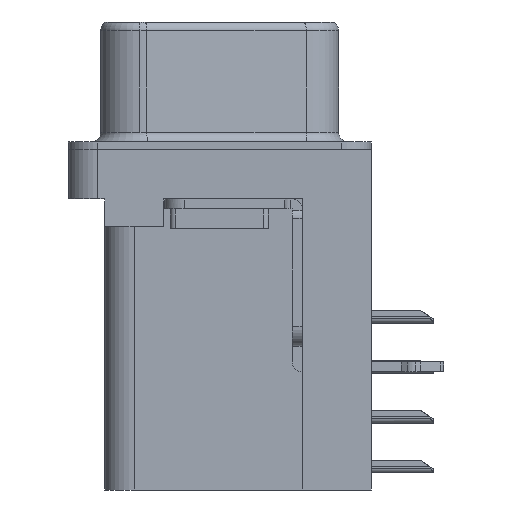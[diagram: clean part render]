
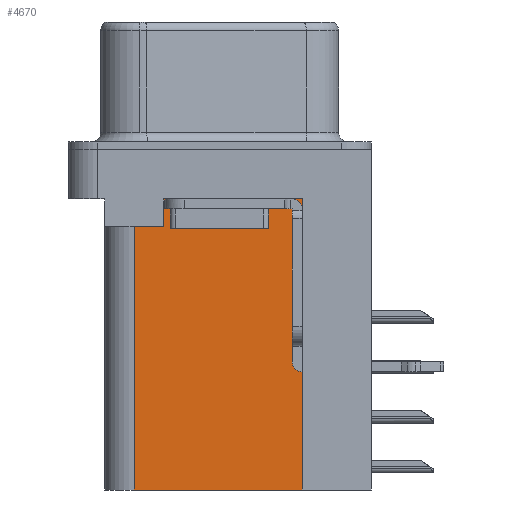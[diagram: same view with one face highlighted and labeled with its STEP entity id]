
A CAD part, left-side view. The second image highlights one B-rep face of the part: STEP entity #4670.
In plain terms, the highlighted planar face has unit normal (-1, 0, 0).
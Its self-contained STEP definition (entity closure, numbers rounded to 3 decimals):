
#1924 = EDGE_CURVE ( 'NONE', #36063, #21664, #15045, .T. ) ;
#2300 = LINE ( 'NONE', #3465, #17706 ) ;
#2521 = DIRECTION ( 'NONE',  ( 0., 1., 0. ) ) ;
#2881 = VERTEX_POINT ( 'NONE', #8026 ) ;
#3465 = CARTESIAN_POINT ( 'NONE',  ( 3.75, 4.35, -17.3 ) ) ;
#4670 = ADVANCED_FACE ( 'NONE', ( #11981 ), #25382, .F. ) ;
#5185 = DIRECTION ( 'NONE',  ( 0., 0., -1. ) ) ;
#5504 = VECTOR ( 'NONE', #10067, 1000. ) ;
#5625 = ORIENTED_EDGE ( 'NONE', *, *, #34127, .F. ) ;
#6606 = VECTOR ( 'NONE', #33735, 1000. ) ;
#7624 = ORIENTED_EDGE ( 'NONE', *, *, #16834, .T. ) ;
#8026 = CARTESIAN_POINT ( 'NONE',  ( 3.75, 2.85, -3.9 ) ) ;
#8383 = VERTEX_POINT ( 'NONE', #8876 ) ;
#8876 = CARTESIAN_POINT ( 'NONE',  ( 3.75, 4.35, -3.9 ) ) ;
#9161 = CARTESIAN_POINT ( 'NONE',  ( 3.75, 0., -3.9 ) ) ;
#9656 = CARTESIAN_POINT ( 'NONE',  ( 3.75, 4.35, -17.3 ) ) ;
#10067 = DIRECTION ( 'NONE',  ( 0., 0., 1. ) ) ;
#10268 = LINE ( 'NONE', #9161, #33986 ) ;
#11162 = VERTEX_POINT ( 'NONE', #9656 ) ;
#11924 = VECTOR ( 'NONE', #40044, 1000. ) ;
#11981 = FACE_OUTER_BOUND ( 'NONE', #33404, .T. ) ;
#13387 = CARTESIAN_POINT ( 'NONE',  ( 3.75, -4.2, -17.3 ) ) ;
#15045 = LINE ( 'NONE', #26072, #11924 ) ;
#16260 = ORIENTED_EDGE ( 'NONE', *, *, #35868, .F. ) ;
#16659 = EDGE_CURVE ( 'NONE', #21664, #2881, #22943, .T. ) ;
#16834 = EDGE_CURVE ( 'NONE', #2881, #8383, #10268, .T. ) ;
#16930 = CARTESIAN_POINT ( 'NONE',  ( 3.75, 2.85, -2.5 ) ) ;
#17706 = VECTOR ( 'NONE', #26108, 1000. ) ;
#21094 = AXIS2_PLACEMENT_3D ( 'NONE', #27506, #24367, #24327 ) ;
#21664 = VERTEX_POINT ( 'NONE', #16930 ) ;
#22943 = LINE ( 'NONE', #27511, #30462 ) ;
#23917 = CARTESIAN_POINT ( 'NONE',  ( 3.75, -4.2, -2.5 ) ) ;
#24327 = DIRECTION ( 'NONE',  ( 0., 1., 0. ) ) ;
#24367 = DIRECTION ( 'NONE',  ( 1., 0., 0. ) ) ;
#24686 = ORIENTED_EDGE ( 'NONE', *, *, #16659, .T. ) ;
#25382 = PLANE ( 'NONE',  #21094 ) ;
#25734 = ORIENTED_EDGE ( 'NONE', *, *, #1924, .T. ) ;
#26072 = CARTESIAN_POINT ( 'NONE',  ( 3.75, -4.2, -2.5 ) ) ;
#26108 = DIRECTION ( 'NONE',  ( 0., 0., 1. ) ) ;
#27015 = CARTESIAN_POINT ( 'NONE',  ( 3.75, -4.2, -17.3 ) ) ;
#27506 = CARTESIAN_POINT ( 'NONE',  ( 3.75, -4.2, -17.3 ) ) ;
#27511 = CARTESIAN_POINT ( 'NONE',  ( 3.75, 2.85, -3.9 ) ) ;
#30462 = VECTOR ( 'NONE', #5185, 1000. ) ;
#30505 = CARTESIAN_POINT ( 'NONE',  ( 3.75, -4.2, -17.3 ) ) ;
#31309 = LINE ( 'NONE', #13387, #5504 ) ;
#33404 = EDGE_LOOP ( 'NONE', ( #25734, #24686, #7624, #16260, #5625, #37117 ) ) ;
#33735 = DIRECTION ( 'NONE',  ( 0., 1., 0. ) ) ;
#33933 = EDGE_CURVE ( 'NONE', #37520, #36063, #31309, .T. ) ;
#33986 = VECTOR ( 'NONE', #2521, 1000. ) ;
#34127 = EDGE_CURVE ( 'NONE', #37520, #11162, #40777, .T. ) ;
#35868 = EDGE_CURVE ( 'NONE', #11162, #8383, #2300, .T. ) ;
#36063 = VERTEX_POINT ( 'NONE', #23917 ) ;
#37117 = ORIENTED_EDGE ( 'NONE', *, *, #33933, .T. ) ;
#37520 = VERTEX_POINT ( 'NONE', #27015 ) ;
#40044 = DIRECTION ( 'NONE',  ( 0., 1., 0. ) ) ;
#40777 = LINE ( 'NONE', #30505, #6606 ) ;
